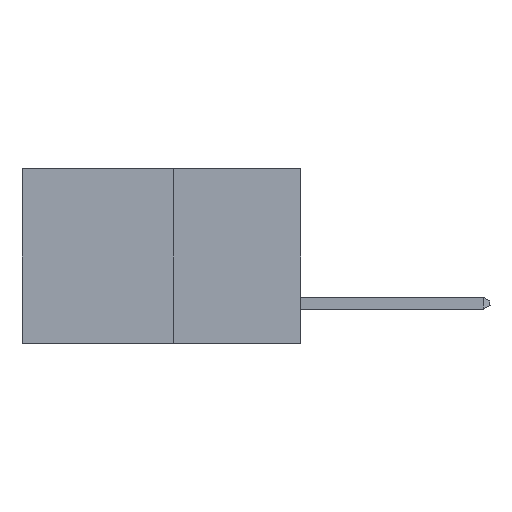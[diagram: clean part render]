
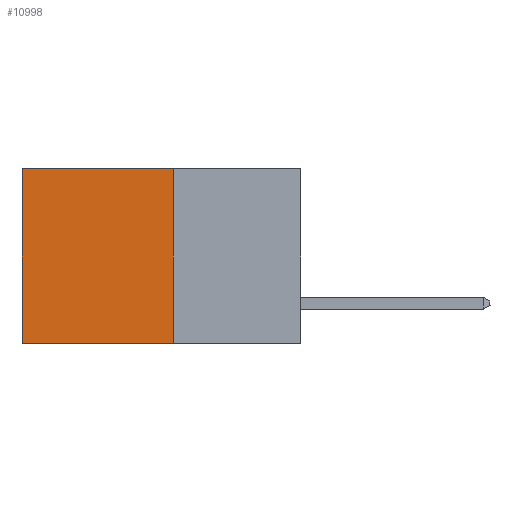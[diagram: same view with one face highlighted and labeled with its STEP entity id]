
A CAD part, left-side view. The second image highlights one B-rep face of the part: STEP entity #10998.
In plain terms, the highlighted planar face has unit normal (-1, 0, 0).
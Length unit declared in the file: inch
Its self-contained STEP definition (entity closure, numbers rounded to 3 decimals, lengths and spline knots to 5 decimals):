
#18 = VERTEX_POINT ( 'NONE', #6783 ) ;
#442 = CARTESIAN_POINT ( 'NONE',  ( 0.277, 0.27, -0.37 ) ) ;
#760 = VERTEX_POINT ( 'NONE', #3655 ) ;
#1075 = VECTOR ( 'NONE', #7480, 39.37008 ) ;
#1483 = PLANE ( 'NONE',  #8877 ) ;
#1554 = CARTESIAN_POINT ( 'NONE',  ( 0.277, 0.27, 0. ) ) ;
#1707 = VERTEX_POINT ( 'NONE', #5228 ) ;
#2204 = DIRECTION ( 'NONE',  ( 0., 0., -1. ) ) ;
#2233 = CARTESIAN_POINT ( 'NONE',  ( 0.277, 0.59, -0.37 ) ) ;
#2509 = DIRECTION ( 'NONE',  ( 1., 0., 0. ) ) ;
#2587 = DIRECTION ( 'NONE',  ( 0., 1., 0. ) ) ;
#2751 = VECTOR ( 'NONE', #9257, 39.37008 ) ;
#2966 = LINE ( 'NONE', #1554, #10835 ) ;
#3062 = LINE ( 'NONE', #8215, #2751 ) ;
#3360 = ORIENTED_EDGE ( 'NONE', *, *, #8856, .F. ) ;
#3655 = CARTESIAN_POINT ( 'NONE',  ( 0.277, 0.59, -0.37 ) ) ;
#4500 = ORIENTED_EDGE ( 'NONE', *, *, #6175, .F. ) ;
#4960 = FACE_OUTER_BOUND ( 'NONE', #6837, .T. ) ;
#5228 = CARTESIAN_POINT ( 'NONE',  ( 0.277, 0.27, 0. ) ) ;
#6175 = EDGE_CURVE ( 'NONE', #18, #760, #11931, .T. ) ;
#6609 = ORIENTED_EDGE ( 'NONE', *, *, #8471, .T. ) ;
#6783 = CARTESIAN_POINT ( 'NONE',  ( 0.277, 0.27, -0.37 ) ) ;
#6837 = EDGE_LOOP ( 'NONE', ( #6609, #4500, #3360, #9171 ) ) ;
#7436 = CARTESIAN_POINT ( 'NONE',  ( 0.277, 0.27, -0.37 ) ) ;
#7480 = DIRECTION ( 'NONE',  ( 0., 1., 0. ) ) ;
#8215 = CARTESIAN_POINT ( 'NONE',  ( 0.277, 0.27, -0.37 ) ) ;
#8471 = EDGE_CURVE ( 'NONE', #12333, #760, #12640, .T. ) ;
#8856 = EDGE_CURVE ( 'NONE', #1707, #18, #3062, .T. ) ;
#8877 = AXIS2_PLACEMENT_3D ( 'NONE', #442, #2509, #9696 ) ;
#9171 = ORIENTED_EDGE ( 'NONE', *, *, #13001, .T. ) ;
#9257 = DIRECTION ( 'NONE',  ( 0., 0., -1. ) ) ;
#9696 = DIRECTION ( 'NONE',  ( 0., 0., -1. ) ) ;
#10835 = VECTOR ( 'NONE', #2587, 39.37008 ) ;
#10998 = ADVANCED_FACE ( 'NONE', ( #4960 ), #1483, .F. ) ;
#11705 = CARTESIAN_POINT ( 'NONE',  ( 0.277, 0.59, 0. ) ) ;
#11931 = LINE ( 'NONE', #7436, #1075 ) ;
#12333 = VERTEX_POINT ( 'NONE', #11705 ) ;
#12640 = LINE ( 'NONE', #2233, #12941 ) ;
#12941 = VECTOR ( 'NONE', #2204, 39.37008 ) ;
#13001 = EDGE_CURVE ( 'NONE', #1707, #12333, #2966, .T. ) ;
